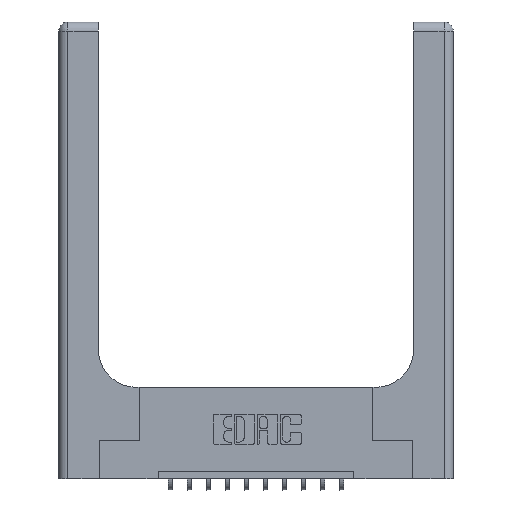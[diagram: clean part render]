
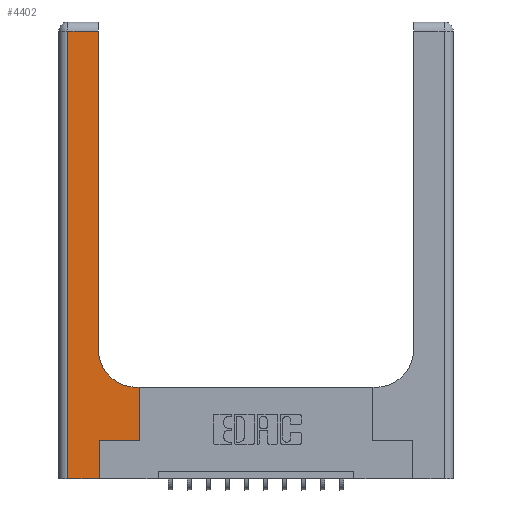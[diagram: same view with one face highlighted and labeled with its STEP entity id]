
A CAD part, top view. The second image highlights one B-rep face of the part: STEP entity #4402.
In plain terms, the highlighted planar face has unit normal (0, 0, 1).
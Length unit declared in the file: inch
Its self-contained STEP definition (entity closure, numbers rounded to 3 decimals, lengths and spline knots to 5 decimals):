
#407 = ORIENTED_EDGE ( 'NONE', *, *, #8371, .T. ) ;
#671 = VERTEX_POINT ( 'NONE', #6302 ) ;
#886 = ORIENTED_EDGE ( 'NONE', *, *, #6925, .T. ) ;
#948 = ORIENTED_EDGE ( 'NONE', *, *, #1272, .T. ) ;
#950 = ORIENTED_EDGE ( 'NONE', *, *, #14503, .T. ) ;
#975 = VECTOR ( 'NONE', #7631, 39.37008 ) ;
#980 = DIRECTION ( 'NONE',  ( 0., 1., 0. ) ) ;
#1074 = DIRECTION ( 'NONE',  ( 0., 0., -1. ) ) ;
#1092 = ORIENTED_EDGE ( 'NONE', *, *, #13182, .T. ) ;
#1272 = EDGE_CURVE ( 'NONE', #6891, #9974, #13714, .T. ) ;
#1331 = VECTOR ( 'NONE', #980, 39.37008 ) ;
#1537 = VECTOR ( 'NONE', #9615, 39.37008 ) ;
#1892 = ORIENTED_EDGE ( 'NONE', *, *, #11566, .T. ) ;
#1988 = EDGE_LOOP ( 'NONE', ( #950, #1092, #5049, #5799, #11528, #407, #886, #948, #1892 ) ) ;
#2090 = VECTOR ( 'NONE', #14389, 39.37008 ) ;
#2179 = CARTESIAN_POINT ( 'NONE',  ( 0.26, 0.85, 0.37 ) ) ;
#2950 = LINE ( 'NONE', #15779, #5846 ) ;
#3346 = LINE ( 'NONE', #8299, #6232 ) ;
#3423 = CARTESIAN_POINT ( 'NONE',  ( 0., 3., 0.37 ) ) ;
#3571 = CARTESIAN_POINT ( 'NONE',  ( 0.51, 0.6, 0.37 ) ) ;
#3966 = CARTESIAN_POINT ( 'NONE',  ( 0.528, 0.25, 0.37 ) ) ;
#4016 = VERTEX_POINT ( 'NONE', #12231 ) ;
#4402 = ADVANCED_FACE ( 'NONE', ( #12761 ), #10699, .F. ) ;
#4635 = LINE ( 'NONE', #7175, #2090 ) ;
#4674 = DIRECTION ( 'NONE',  ( -1., 0., 0. ) ) ;
#5049 = ORIENTED_EDGE ( 'NONE', *, *, #12395, .T. ) ;
#5052 = LINE ( 'NONE', #15542, #1331 ) ;
#5340 = VERTEX_POINT ( 'NONE', #8250 ) ;
#5563 = AXIS2_PLACEMENT_3D ( 'NONE', #3423, #11898, #4674 ) ;
#5799 = ORIENTED_EDGE ( 'NONE', *, *, #8241, .T. ) ;
#5846 = VECTOR ( 'NONE', #6197, 39.37008 ) ;
#6197 = DIRECTION ( 'NONE',  ( 1., 0., 0. ) ) ;
#6232 = VECTOR ( 'NONE', #14296, 39.37008 ) ;
#6302 = CARTESIAN_POINT ( 'NONE',  ( 0.06, 0., 0.37 ) ) ;
#6368 = AXIS2_PLACEMENT_3D ( 'NONE', #8437, #1074, #9638 ) ;
#6410 = VECTOR ( 'NONE', #6862, 39.37008 ) ;
#6421 = CARTESIAN_POINT ( 'NONE',  ( 0.265, 0.25, 0.37 ) ) ;
#6862 = DIRECTION ( 'NONE',  ( -1., 0., 0. ) ) ;
#6891 = VERTEX_POINT ( 'NONE', #11175 ) ;
#6925 = EDGE_CURVE ( 'NONE', #9522, #6891, #7587, .T. ) ;
#7175 = CARTESIAN_POINT ( 'NONE',  ( 0.265, 0., 0.37 ) ) ;
#7203 = VECTOR ( 'NONE', #10009, 39.37008 ) ;
#7544 = LINE ( 'NONE', #6421, #975 ) ;
#7587 = LINE ( 'NONE', #3966, #7203 ) ;
#7631 = DIRECTION ( 'NONE',  ( 1., 0., 0. ) ) ;
#8241 = EDGE_CURVE ( 'NONE', #671, #12717, #2950, .T. ) ;
#8250 = CARTESIAN_POINT ( 'NONE',  ( 0.06, 2.94, 0.37 ) ) ;
#8299 = CARTESIAN_POINT ( 'NONE',  ( 0.06, 3., 0.37 ) ) ;
#8361 = VERTEX_POINT ( 'NONE', #10001 ) ;
#8371 = EDGE_CURVE ( 'NONE', #8361, #9522, #7544, .T. ) ;
#8437 = CARTESIAN_POINT ( 'NONE',  ( 0.51, 0.85, 0.37 ) ) ;
#8751 = VERTEX_POINT ( 'NONE', #2179 ) ;
#9522 = VERTEX_POINT ( 'NONE', #11125 ) ;
#9615 = DIRECTION ( 'NONE',  ( -1., 0., 0. ) ) ;
#9638 = DIRECTION ( 'NONE',  ( 1., 0., 0. ) ) ;
#9736 = CARTESIAN_POINT ( 'NONE',  ( 0.26, 0.6, 0.37 ) ) ;
#9974 = VERTEX_POINT ( 'NONE', #3571 ) ;
#10001 = CARTESIAN_POINT ( 'NONE',  ( 0.265, 0.25, 0.37 ) ) ;
#10009 = DIRECTION ( 'NONE',  ( 0., 1., 0. ) ) ;
#10699 = PLANE ( 'NONE',  #5563 ) ;
#11125 = CARTESIAN_POINT ( 'NONE',  ( 0.528, 0.25, 0.37 ) ) ;
#11175 = CARTESIAN_POINT ( 'NONE',  ( 0.528, 0.6, 0.37 ) ) ;
#11307 = CARTESIAN_POINT ( 'NONE',  ( 0.265, 0., 0.37 ) ) ;
#11528 = ORIENTED_EDGE ( 'NONE', *, *, #15014, .T. ) ;
#11566 = EDGE_CURVE ( 'NONE', #9974, #8751, #12867, .T. ) ;
#11898 = DIRECTION ( 'NONE',  ( 0., 0., -1. ) ) ;
#12047 = LINE ( 'NONE', #14066, #6410 ) ;
#12231 = CARTESIAN_POINT ( 'NONE',  ( 0.26, 2.94, 0.37 ) ) ;
#12395 = EDGE_CURVE ( 'NONE', #5340, #671, #3346, .T. ) ;
#12717 = VERTEX_POINT ( 'NONE', #11307 ) ;
#12761 = FACE_OUTER_BOUND ( 'NONE', #1988, .T. ) ;
#12867 = CIRCLE ( 'NONE', #6368, 0.25 ) ;
#13182 = EDGE_CURVE ( 'NONE', #4016, #5340, #12047, .T. ) ;
#13714 = LINE ( 'NONE', #9736, #1537 ) ;
#14066 = CARTESIAN_POINT ( 'NONE',  ( 0., 2.94, 0.37 ) ) ;
#14296 = DIRECTION ( 'NONE',  ( 0., -1., 0. ) ) ;
#14389 = DIRECTION ( 'NONE',  ( 0., 1., 0. ) ) ;
#14503 = EDGE_CURVE ( 'NONE', #8751, #4016, #5052, .T. ) ;
#15014 = EDGE_CURVE ( 'NONE', #12717, #8361, #4635, .T. ) ;
#15542 = CARTESIAN_POINT ( 'NONE',  ( 0.26, 3., 0.37 ) ) ;
#15779 = CARTESIAN_POINT ( 'NONE',  ( 0., 0., 0.37 ) ) ;
